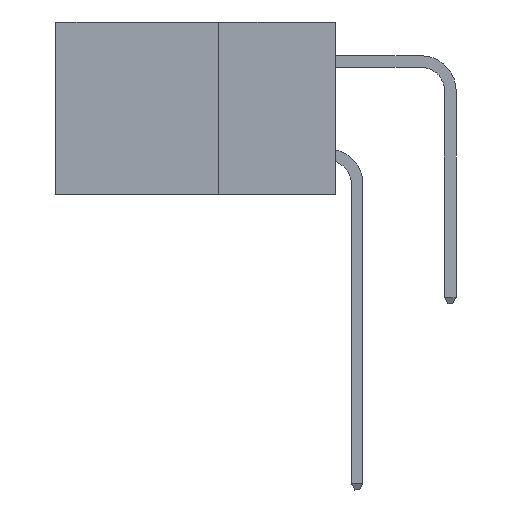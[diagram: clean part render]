
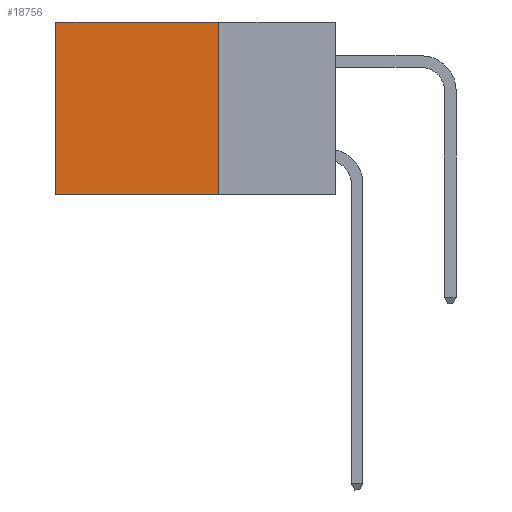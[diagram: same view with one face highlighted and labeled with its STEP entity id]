
A CAD part, left-side view. The second image highlights one B-rep face of the part: STEP entity #18756.
In plain terms, the highlighted planar face has unit normal (-1, 0, 0).
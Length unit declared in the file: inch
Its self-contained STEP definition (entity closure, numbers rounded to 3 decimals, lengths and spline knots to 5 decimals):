
#125 = ORIENTED_EDGE ( 'NONE', *, *, #4654, .F. ) ;
#326 = CARTESIAN_POINT ( 'NONE',  ( 0.2875, 0.25, -0.37 ) ) ;
#390 = DIRECTION ( 'NONE',  ( 1., 0., 0. ) ) ;
#1731 = CARTESIAN_POINT ( 'NONE',  ( 0.2875, 0.6, 0. ) ) ;
#1952 = ORIENTED_EDGE ( 'NONE', *, *, #3452, .T. ) ;
#3123 = VECTOR ( 'NONE', #12909, 39.37008 ) ;
#3452 = EDGE_CURVE ( 'NONE', #9842, #19418, #7926, .T. ) ;
#3690 = VECTOR ( 'NONE', #14617, 39.37008 ) ;
#4654 = EDGE_CURVE ( 'NONE', #7804, #8813, #8823, .T. ) ;
#4724 = CARTESIAN_POINT ( 'NONE',  ( 0.2875, 0.25, -0.37 ) ) ;
#5175 = CARTESIAN_POINT ( 'NONE',  ( 0.2875, 0.6, 0. ) ) ;
#5372 = ORIENTED_EDGE ( 'NONE', *, *, #15516, .F. ) ;
#5526 = CARTESIAN_POINT ( 'NONE',  ( 0.2875, 0.6, -0.37 ) ) ;
#7250 = DIRECTION ( 'NONE',  ( 0., 0., -1. ) ) ;
#7804 = VERTEX_POINT ( 'NONE', #4724 ) ;
#7926 = LINE ( 'NONE', #11397, #3123 ) ;
#8363 = PLANE ( 'NONE',  #17438 ) ;
#8448 = LINE ( 'NONE', #5175, #3690 ) ;
#8699 = EDGE_CURVE ( 'NONE', #19418, #8813, #8448, .T. ) ;
#8813 = VERTEX_POINT ( 'NONE', #5526 ) ;
#8823 = LINE ( 'NONE', #326, #12440 ) ;
#8863 = EDGE_LOOP ( 'NONE', ( #15979, #125, #5372, #1952 ) ) ;
#8878 = VECTOR ( 'NONE', #7250, 39.37008 ) ;
#9842 = VERTEX_POINT ( 'NONE', #10585 ) ;
#10585 = CARTESIAN_POINT ( 'NONE',  ( 0.2875, 0.25, 0. ) ) ;
#11397 = CARTESIAN_POINT ( 'NONE',  ( 0.2875, 0.25, 0. ) ) ;
#11487 = DIRECTION ( 'NONE',  ( 0., 0., -1. ) ) ;
#12440 = VECTOR ( 'NONE', #12938, 39.37008 ) ;
#12909 = DIRECTION ( 'NONE',  ( 0., 1., 0. ) ) ;
#12938 = DIRECTION ( 'NONE',  ( 0., 1., 0. ) ) ;
#14617 = DIRECTION ( 'NONE',  ( 0., 0., -1. ) ) ;
#15516 = EDGE_CURVE ( 'NONE', #9842, #7804, #16201, .T. ) ;
#15979 = ORIENTED_EDGE ( 'NONE', *, *, #8699, .T. ) ;
#16201 = LINE ( 'NONE', #16590, #8878 ) ;
#16590 = CARTESIAN_POINT ( 'NONE',  ( 0.2875, 0.25, 0. ) ) ;
#17438 = AXIS2_PLACEMENT_3D ( 'NONE', #19253, #390, #11487 ) ;
#18751 = FACE_OUTER_BOUND ( 'NONE', #8863, .T. ) ;
#18756 = ADVANCED_FACE ( 'NONE', ( #18751 ), #8363, .F. ) ;
#19253 = CARTESIAN_POINT ( 'NONE',  ( 0.2875, 0.25, 0. ) ) ;
#19418 = VERTEX_POINT ( 'NONE', #1731 ) ;
